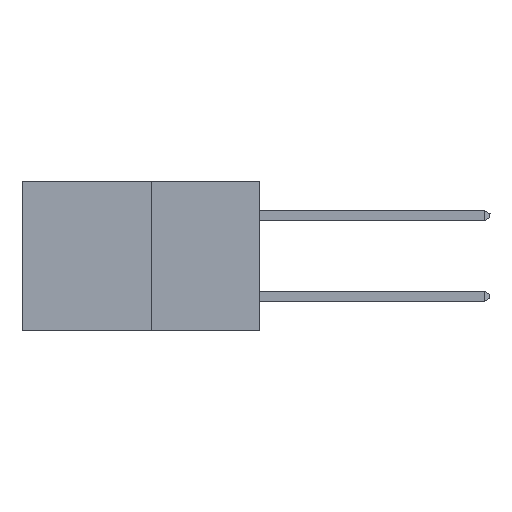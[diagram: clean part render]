
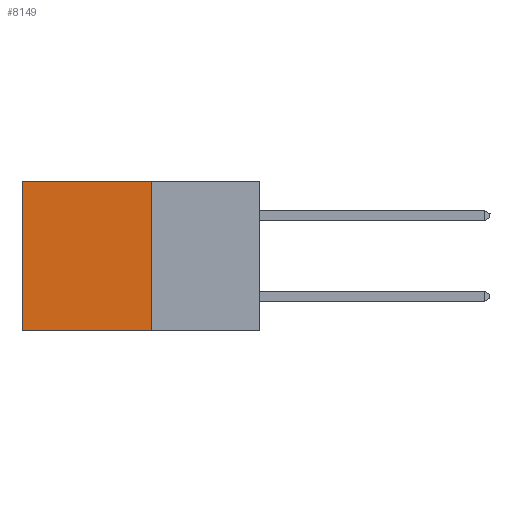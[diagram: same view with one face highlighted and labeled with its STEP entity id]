
A CAD part, left-side view. The second image highlights one B-rep face of the part: STEP entity #8149.
In plain terms, the highlighted planar face has unit normal (-1, 0, 0).
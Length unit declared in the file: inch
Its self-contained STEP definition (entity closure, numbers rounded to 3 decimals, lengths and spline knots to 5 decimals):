
#325 = CARTESIAN_POINT ( 'NONE',  ( 0.277, 0.27, -0.37 ) ) ;
#3474 = EDGE_LOOP ( 'NONE', ( #11506, #9481, #13411, #7120 ) ) ;
#3612 = CARTESIAN_POINT ( 'NONE',  ( 0.277, 0.27, -0.37 ) ) ;
#3731 = EDGE_CURVE ( 'NONE', #13448, #13224, #8893, .T. ) ;
#3973 = DIRECTION ( 'NONE',  ( 0., 0., -1. ) ) ;
#4079 = DIRECTION ( 'NONE',  ( 1., 0., 0. ) ) ;
#4679 = VECTOR ( 'NONE', #11950, 39.37008 ) ;
#5103 = LINE ( 'NONE', #10631, #4679 ) ;
#5454 = VECTOR ( 'NONE', #12863, 39.37008 ) ;
#7120 = ORIENTED_EDGE ( 'NONE', *, *, #16749, .T. ) ;
#7405 = CARTESIAN_POINT ( 'NONE',  ( 0.277, 0.27, 0. ) ) ;
#7662 = EDGE_CURVE ( 'NONE', #13224, #15307, #12883, .T. ) ;
#8147 = DIRECTION ( 'NONE',  ( 0., 1., 0. ) ) ;
#8149 = ADVANCED_FACE ( 'NONE', ( #11614 ), #9275, .F. ) ;
#8893 = LINE ( 'NONE', #3612, #15775 ) ;
#8969 = CARTESIAN_POINT ( 'NONE',  ( 0.277, 0.59, -0.37 ) ) ;
#9275 = PLANE ( 'NONE',  #9438 ) ;
#9438 = AXIS2_PLACEMENT_3D ( 'NONE', #14459, #4079, #13223 ) ;
#9481 = ORIENTED_EDGE ( 'NONE', *, *, #7662, .F. ) ;
#10631 = CARTESIAN_POINT ( 'NONE',  ( 0.277, 0.27, 0. ) ) ;
#11109 = VERTEX_POINT ( 'NONE', #13869 ) ;
#11506 = ORIENTED_EDGE ( 'NONE', *, *, #11981, .T. ) ;
#11614 = FACE_OUTER_BOUND ( 'NONE', #3474, .T. ) ;
#11950 = DIRECTION ( 'NONE',  ( 0., 1., 0. ) ) ;
#11981 = EDGE_CURVE ( 'NONE', #11109, #15307, #12383, .T. ) ;
#12383 = LINE ( 'NONE', #8969, #5454 ) ;
#12863 = DIRECTION ( 'NONE',  ( 0., 0., -1. ) ) ;
#12883 = LINE ( 'NONE', #325, #15855 ) ;
#13223 = DIRECTION ( 'NONE',  ( 0., 0., -1. ) ) ;
#13224 = VERTEX_POINT ( 'NONE', #15976 ) ;
#13411 = ORIENTED_EDGE ( 'NONE', *, *, #3731, .F. ) ;
#13448 = VERTEX_POINT ( 'NONE', #7405 ) ;
#13869 = CARTESIAN_POINT ( 'NONE',  ( 0.277, 0.59, 0. ) ) ;
#14459 = CARTESIAN_POINT ( 'NONE',  ( 0.277, 0.27, -0.37 ) ) ;
#15109 = CARTESIAN_POINT ( 'NONE',  ( 0.277, 0.59, -0.37 ) ) ;
#15307 = VERTEX_POINT ( 'NONE', #15109 ) ;
#15775 = VECTOR ( 'NONE', #3973, 39.37008 ) ;
#15855 = VECTOR ( 'NONE', #8147, 39.37008 ) ;
#15976 = CARTESIAN_POINT ( 'NONE',  ( 0.277, 0.27, -0.37 ) ) ;
#16749 = EDGE_CURVE ( 'NONE', #13448, #11109, #5103, .T. ) ;
